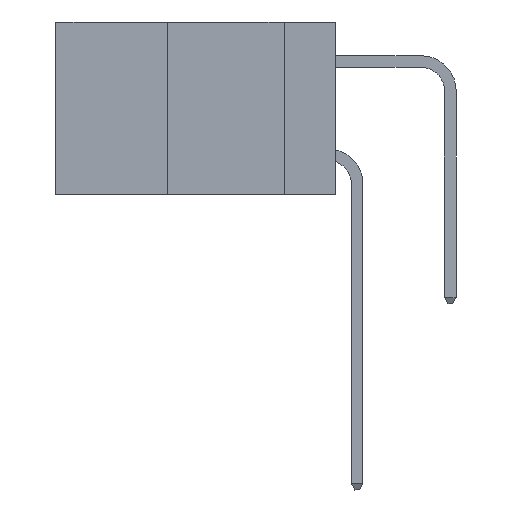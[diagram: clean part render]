
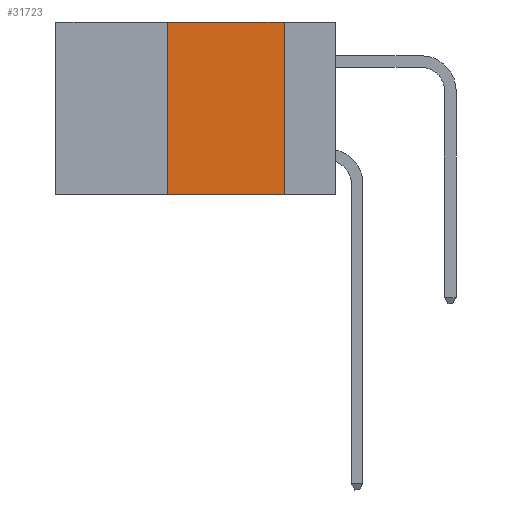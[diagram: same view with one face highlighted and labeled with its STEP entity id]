
A CAD part, left-side view. The second image highlights one B-rep face of the part: STEP entity #31723.
In plain terms, the highlighted planar face has unit normal (-1, 0, 0).
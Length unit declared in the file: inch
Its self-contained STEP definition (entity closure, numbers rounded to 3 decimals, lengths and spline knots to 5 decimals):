
#2854 = VECTOR ( 'NONE', #10925, 39.37008 ) ;
#4051 = EDGE_CURVE ( 'NONE', #20938, #15531, #22028, .T. ) ;
#5598 = CARTESIAN_POINT ( 'NONE',  ( 0., 0.36, 0. ) ) ;
#5818 = EDGE_LOOP ( 'NONE', ( #7751, #24914, #30925, #6224 ) ) ;
#6224 = ORIENTED_EDGE ( 'NONE', *, *, #26555, .T. ) ;
#7094 = EDGE_CURVE ( 'NONE', #15531, #16884, #29671, .T. ) ;
#7751 = ORIENTED_EDGE ( 'NONE', *, *, #30050, .F. ) ;
#8148 = CARTESIAN_POINT ( 'NONE',  ( 0., 0.11, 0. ) ) ;
#10317 = CARTESIAN_POINT ( 'NONE',  ( 0., 0.6, 0. ) ) ;
#10925 = DIRECTION ( 'NONE',  ( 0., -1., 0. ) ) ;
#11316 = VECTOR ( 'NONE', #11426, 39.37008 ) ;
#11426 = DIRECTION ( 'NONE',  ( 0., 0., -1. ) ) ;
#12330 = CARTESIAN_POINT ( 'NONE',  ( 0., 0.11, 0. ) ) ;
#13548 = DIRECTION ( 'NONE',  ( 0., 0., -1. ) ) ;
#13736 = FACE_OUTER_BOUND ( 'NONE', #5818, .T. ) ;
#15531 = VERTEX_POINT ( 'NONE', #5598 ) ;
#15547 = CARTESIAN_POINT ( 'NONE',  ( 0., 0.6, -0.37 ) ) ;
#15620 = DIRECTION ( 'NONE',  ( 0., 0., 1. ) ) ;
#16884 = VERTEX_POINT ( 'NONE', #12330 ) ;
#20886 = LINE ( 'NONE', #8148, #11316 ) ;
#20938 = VERTEX_POINT ( 'NONE', #21239 ) ;
#21239 = CARTESIAN_POINT ( 'NONE',  ( 0., 0.36, -0.37 ) ) ;
#22028 = LINE ( 'NONE', #34827, #40006 ) ;
#23391 = VERTEX_POINT ( 'NONE', #39511 ) ;
#24914 = ORIENTED_EDGE ( 'NONE', *, *, #7094, .F. ) ;
#26342 = PLANE ( 'NONE',  #30040 ) ;
#26555 = EDGE_CURVE ( 'NONE', #20938, #23391, #33065, .T. ) ;
#29671 = LINE ( 'NONE', #33369, #2854 ) ;
#30040 = AXIS2_PLACEMENT_3D ( 'NONE', #10317, #32762, #13548 ) ;
#30050 = EDGE_CURVE ( 'NONE', #16884, #23391, #20886, .T. ) ;
#30925 = ORIENTED_EDGE ( 'NONE', *, *, #4051, .F. ) ;
#31723 = ADVANCED_FACE ( 'NONE', ( #13736 ), #26342, .F. ) ;
#32065 = VECTOR ( 'NONE', #34750, 39.37008 ) ;
#32762 = DIRECTION ( 'NONE',  ( 1., 0., 0. ) ) ;
#33065 = LINE ( 'NONE', #15547, #32065 ) ;
#33369 = CARTESIAN_POINT ( 'NONE',  ( 0., 0.6, 0. ) ) ;
#34750 = DIRECTION ( 'NONE',  ( 0., -1., 0. ) ) ;
#34827 = CARTESIAN_POINT ( 'NONE',  ( 0., 0.36, 0. ) ) ;
#39511 = CARTESIAN_POINT ( 'NONE',  ( 0., 0.11, -0.37 ) ) ;
#40006 = VECTOR ( 'NONE', #15620, 39.37008 ) ;
